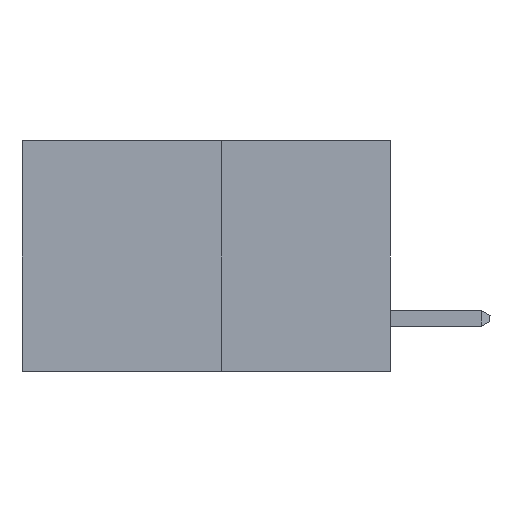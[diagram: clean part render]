
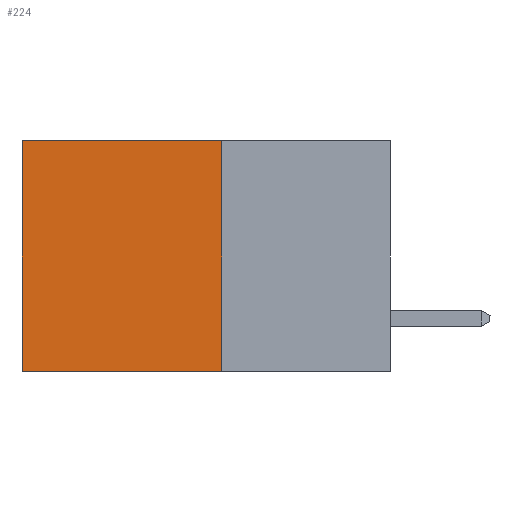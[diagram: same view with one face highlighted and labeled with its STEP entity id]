
A CAD part, left-side view. The second image highlights one B-rep face of the part: STEP entity #224.
In plain terms, the highlighted planar face has unit normal (-1, 0, 0).
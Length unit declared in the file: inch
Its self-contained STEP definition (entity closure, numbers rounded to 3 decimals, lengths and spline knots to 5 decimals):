
#106 = CARTESIAN_POINT ( 'NONE',  ( 0.277, 0.27, -0.37 ) ) ;
#202 = VECTOR ( 'NONE', #8746, 39.37008 ) ;
#224 = ADVANCED_FACE ( 'NONE', ( #3652 ), #8650, .F. ) ;
#362 = DIRECTION ( 'NONE',  ( 0., 1., 0. ) ) ;
#407 = ORIENTED_EDGE ( 'NONE', *, *, #1262, .F. ) ;
#1028 = LINE ( 'NONE', #7190, #11869 ) ;
#1144 = LINE ( 'NONE', #6763, #8939 ) ;
#1262 = EDGE_CURVE ( 'NONE', #4783, #5808, #13038, .T. ) ;
#2097 = VERTEX_POINT ( 'NONE', #9976 ) ;
#2998 = ORIENTED_EDGE ( 'NONE', *, *, #7663, .T. ) ;
#3375 = EDGE_CURVE ( 'NONE', #4783, #2097, #1028, .T. ) ;
#3652 = FACE_OUTER_BOUND ( 'NONE', #6616, .T. ) ;
#4783 = VERTEX_POINT ( 'NONE', #8291 ) ;
#4843 = VECTOR ( 'NONE', #5259, 39.37008 ) ;
#5259 = DIRECTION ( 'NONE',  ( 0., 0., -1. ) ) ;
#5532 = CARTESIAN_POINT ( 'NONE',  ( 0.277, 0.59, -0.37 ) ) ;
#5736 = ORIENTED_EDGE ( 'NONE', *, *, #6592, .F. ) ;
#5808 = VERTEX_POINT ( 'NONE', #106 ) ;
#6310 = DIRECTION ( 'NONE',  ( 1., 0., 0. ) ) ;
#6592 = EDGE_CURVE ( 'NONE', #5808, #8923, #1144, .T. ) ;
#6616 = EDGE_LOOP ( 'NONE', ( #2998, #5736, #407, #11625 ) ) ;
#6763 = CARTESIAN_POINT ( 'NONE',  ( 0.277, 0.27, -0.37 ) ) ;
#7190 = CARTESIAN_POINT ( 'NONE',  ( 0.277, 0.27, 0. ) ) ;
#7292 = DIRECTION ( 'NONE',  ( 0., 0., -1. ) ) ;
#7663 = EDGE_CURVE ( 'NONE', #2097, #8923, #11458, .T. ) ;
#7671 = CARTESIAN_POINT ( 'NONE',  ( 0.277, 0.59, -0.37 ) ) ;
#8291 = CARTESIAN_POINT ( 'NONE',  ( 0.277, 0.27, 0. ) ) ;
#8634 = CARTESIAN_POINT ( 'NONE',  ( 0.277, 0.27, -0.37 ) ) ;
#8650 = PLANE ( 'NONE',  #11165 ) ;
#8746 = DIRECTION ( 'NONE',  ( 0., 0., -1. ) ) ;
#8923 = VERTEX_POINT ( 'NONE', #7671 ) ;
#8939 = VECTOR ( 'NONE', #11936, 39.37008 ) ;
#9976 = CARTESIAN_POINT ( 'NONE',  ( 0.277, 0.59, 0. ) ) ;
#10956 = CARTESIAN_POINT ( 'NONE',  ( 0.277, 0.27, -0.37 ) ) ;
#11165 = AXIS2_PLACEMENT_3D ( 'NONE', #8634, #6310, #7292 ) ;
#11458 = LINE ( 'NONE', #5532, #202 ) ;
#11625 = ORIENTED_EDGE ( 'NONE', *, *, #3375, .T. ) ;
#11869 = VECTOR ( 'NONE', #362, 39.37008 ) ;
#11936 = DIRECTION ( 'NONE',  ( 0., 1., 0. ) ) ;
#13038 = LINE ( 'NONE', #10956, #4843 ) ;
